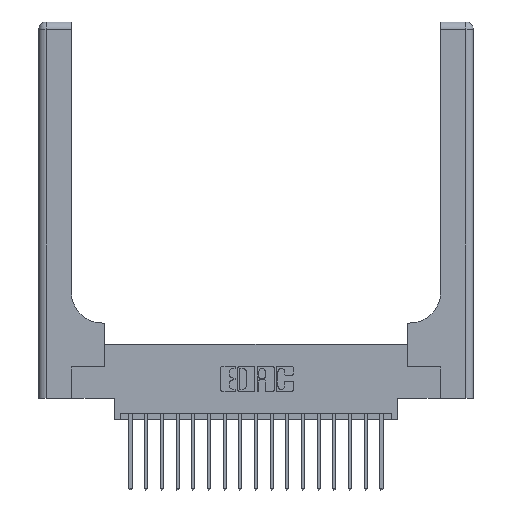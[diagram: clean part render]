
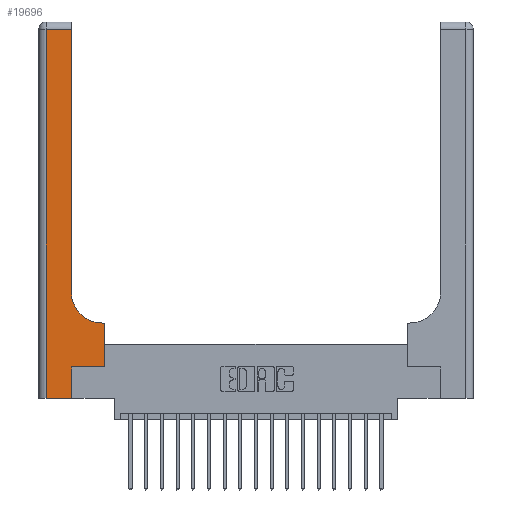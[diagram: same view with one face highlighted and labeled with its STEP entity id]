
A CAD part, top view. The second image highlights one B-rep face of the part: STEP entity #19696.
In plain terms, the highlighted planar face has unit normal (0, 0, 1).
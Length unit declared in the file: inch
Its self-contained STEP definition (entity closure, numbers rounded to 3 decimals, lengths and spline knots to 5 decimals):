
#10 = CARTESIAN_POINT ( 'NONE',  ( 0.26, 3., 0.37 ) ) ;
#260 = EDGE_CURVE ( 'NONE', #8092, #7181, #11623, .T. ) ;
#908 = DIRECTION ( 'NONE',  ( 0., 1., 0. ) ) ;
#1243 = LINE ( 'NONE', #10450, #19094 ) ;
#1311 = CARTESIAN_POINT ( 'NONE',  ( 0., 0., 0.37 ) ) ;
#1327 = VERTEX_POINT ( 'NONE', #16824 ) ;
#1523 = VECTOR ( 'NONE', #19641, 39.37008 ) ;
#1807 = CARTESIAN_POINT ( 'NONE',  ( 0.265, 0.25, 0.37 ) ) ;
#2191 = ORIENTED_EDGE ( 'NONE', *, *, #12781, .T. ) ;
#2787 = PLANE ( 'NONE',  #5135 ) ;
#2840 = VECTOR ( 'NONE', #14762, 39.37008 ) ;
#3283 = DIRECTION ( 'NONE',  ( 0., -1., 0. ) ) ;
#3791 = DIRECTION ( 'NONE',  ( 1., 0., 0. ) ) ;
#4584 = CARTESIAN_POINT ( 'NONE',  ( 0.265, 0.25, 0.37 ) ) ;
#4741 = DIRECTION ( 'NONE',  ( -1., 0., 0. ) ) ;
#5135 = AXIS2_PLACEMENT_3D ( 'NONE', #17091, #16689, #4741 ) ;
#5335 = CARTESIAN_POINT ( 'NONE',  ( 0.26, 0.85, 0.37 ) ) ;
#5731 = ORIENTED_EDGE ( 'NONE', *, *, #14063, .T. ) ;
#6427 = CARTESIAN_POINT ( 'NONE',  ( 0.51, 0.85, 0.37 ) ) ;
#7181 = VERTEX_POINT ( 'NONE', #12472 ) ;
#7331 = CARTESIAN_POINT ( 'NONE',  ( 0.06, 0., 0.37 ) ) ;
#7809 = CARTESIAN_POINT ( 'NONE',  ( 0.26, 2.94, 0.37 ) ) ;
#8092 = VERTEX_POINT ( 'NONE', #7809 ) ;
#8879 = LINE ( 'NONE', #1311, #15575 ) ;
#8962 = ORIENTED_EDGE ( 'NONE', *, *, #19430, .T. ) ;
#9462 = VERTEX_POINT ( 'NONE', #5335 ) ;
#9759 = LINE ( 'NONE', #4584, #16162 ) ;
#9861 = EDGE_CURVE ( 'NONE', #18014, #13205, #16540, .T. ) ;
#10021 = VECTOR ( 'NONE', #14196, 39.37008 ) ;
#10450 = CARTESIAN_POINT ( 'NONE',  ( 0.265, 0., 0.37 ) ) ;
#10515 = LINE ( 'NONE', #16940, #1523 ) ;
#10731 = DIRECTION ( 'NONE',  ( 1., 0., 0. ) ) ;
#10764 = DIRECTION ( 'NONE',  ( 0., 1., 0. ) ) ;
#11623 = LINE ( 'NONE', #17728, #2840 ) ;
#12450 = VECTOR ( 'NONE', #908, 39.37008 ) ;
#12472 = CARTESIAN_POINT ( 'NONE',  ( 0.06, 2.94, 0.37 ) ) ;
#12781 = EDGE_CURVE ( 'NONE', #16476, #9462, #13524, .T. ) ;
#13205 = VERTEX_POINT ( 'NONE', #15082 ) ;
#13283 = CARTESIAN_POINT ( 'NONE',  ( 0.528, 0.25, 0.37 ) ) ;
#13523 = ORIENTED_EDGE ( 'NONE', *, *, #9861, .T. ) ;
#13524 = CIRCLE ( 'NONE', #16150, 0.25 ) ;
#14023 = FACE_OUTER_BOUND ( 'NONE', #18413, .T. ) ;
#14035 = ORIENTED_EDGE ( 'NONE', *, *, #15036, .T. ) ;
#14063 = EDGE_CURVE ( 'NONE', #9462, #8092, #14395, .T. ) ;
#14196 = DIRECTION ( 'NONE',  ( 0., 1., 0. ) ) ;
#14395 = LINE ( 'NONE', #10, #10021 ) ;
#14402 = VERTEX_POINT ( 'NONE', #1807 ) ;
#14508 = LINE ( 'NONE', #18943, #14835 ) ;
#14762 = DIRECTION ( 'NONE',  ( -1., 0., 0. ) ) ;
#14835 = VECTOR ( 'NONE', #3283, 39.37008 ) ;
#15036 = EDGE_CURVE ( 'NONE', #1327, #14402, #1243, .T. ) ;
#15082 = CARTESIAN_POINT ( 'NONE',  ( 0.528, 0.6, 0.37 ) ) ;
#15136 = ORIENTED_EDGE ( 'NONE', *, *, #19219, .T. ) ;
#15180 = EDGE_CURVE ( 'NONE', #7181, #17364, #14508, .T. ) ;
#15575 = VECTOR ( 'NONE', #10731, 39.37008 ) ;
#15795 = DIRECTION ( 'NONE',  ( 1., 0., 0. ) ) ;
#16150 = AXIS2_PLACEMENT_3D ( 'NONE', #6427, #17779, #3791 ) ;
#16162 = VECTOR ( 'NONE', #15795, 39.37008 ) ;
#16476 = VERTEX_POINT ( 'NONE', #18133 ) ;
#16540 = LINE ( 'NONE', #13283, #12450 ) ;
#16689 = DIRECTION ( 'NONE',  ( 0., 0., -1. ) ) ;
#16824 = CARTESIAN_POINT ( 'NONE',  ( 0.265, 0., 0.37 ) ) ;
#16830 = ORIENTED_EDGE ( 'NONE', *, *, #19205, .T. ) ;
#16940 = CARTESIAN_POINT ( 'NONE',  ( 0.26, 0.6, 0.37 ) ) ;
#17091 = CARTESIAN_POINT ( 'NONE',  ( 0., 3., 0.37 ) ) ;
#17364 = VERTEX_POINT ( 'NONE', #7331 ) ;
#17461 = ORIENTED_EDGE ( 'NONE', *, *, #15180, .T. ) ;
#17728 = CARTESIAN_POINT ( 'NONE',  ( 0., 2.94, 0.37 ) ) ;
#17779 = DIRECTION ( 'NONE',  ( 0., 0., -1. ) ) ;
#18014 = VERTEX_POINT ( 'NONE', #18888 ) ;
#18133 = CARTESIAN_POINT ( 'NONE',  ( 0.51, 0.6, 0.37 ) ) ;
#18413 = EDGE_LOOP ( 'NONE', ( #5731, #19224, #17461, #15136, #14035, #8962, #13523, #16830, #2191 ) ) ;
#18888 = CARTESIAN_POINT ( 'NONE',  ( 0.528, 0.25, 0.37 ) ) ;
#18943 = CARTESIAN_POINT ( 'NONE',  ( 0.06, 3., 0.37 ) ) ;
#19094 = VECTOR ( 'NONE', #10764, 39.37008 ) ;
#19205 = EDGE_CURVE ( 'NONE', #13205, #16476, #10515, .T. ) ;
#19219 = EDGE_CURVE ( 'NONE', #17364, #1327, #8879, .T. ) ;
#19224 = ORIENTED_EDGE ( 'NONE', *, *, #260, .T. ) ;
#19430 = EDGE_CURVE ( 'NONE', #14402, #18014, #9759, .T. ) ;
#19641 = DIRECTION ( 'NONE',  ( -1., 0., 0. ) ) ;
#19696 = ADVANCED_FACE ( 'NONE', ( #14023 ), #2787, .F. ) ;
